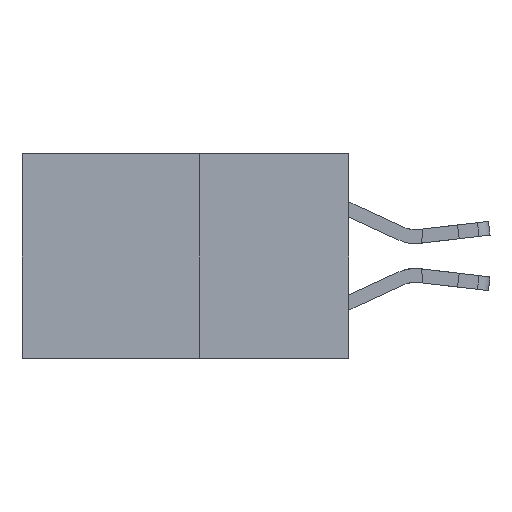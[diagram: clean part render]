
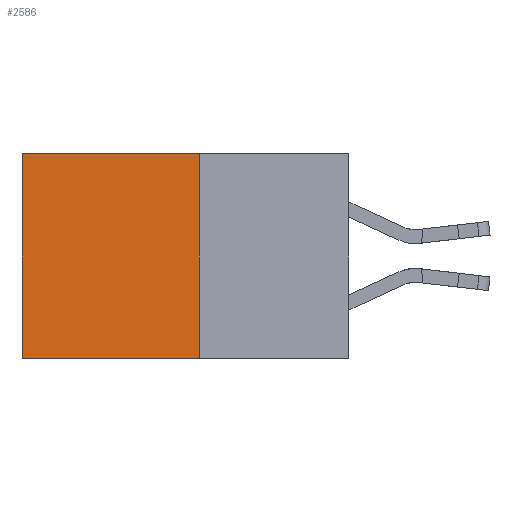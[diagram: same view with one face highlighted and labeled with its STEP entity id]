
A CAD part, left-side view. The second image highlights one B-rep face of the part: STEP entity #2586.
In plain terms, the highlighted planar face has unit normal (-1, 0, 0).
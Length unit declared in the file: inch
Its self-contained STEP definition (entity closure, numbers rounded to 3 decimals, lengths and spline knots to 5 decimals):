
#629 = VERTEX_POINT ( 'NONE', #17003 ) ;
#1297 = DIRECTION ( 'NONE',  ( 0., 1., 0. ) ) ;
#1304 = ORIENTED_EDGE ( 'NONE', *, *, #14577, .T. ) ;
#2586 = ADVANCED_FACE ( 'NONE', ( #15125 ), #15491, .F. ) ;
#3340 = DIRECTION ( 'NONE',  ( 0., 0., -1. ) ) ;
#4838 = CARTESIAN_POINT ( 'NONE',  ( 0.277, 0.27, -0.37 ) ) ;
#7273 = CARTESIAN_POINT ( 'NONE',  ( 0.277, 0.27, -0.37 ) ) ;
#7343 = CARTESIAN_POINT ( 'NONE',  ( 0.277, 0.27, -0.37 ) ) ;
#7575 = EDGE_LOOP ( 'NONE', ( #1304, #23782, #24916, #26746 ) ) ;
#7946 = CARTESIAN_POINT ( 'NONE',  ( 0.277, 0.59, -0.37 ) ) ;
#9758 = VECTOR ( 'NONE', #11988, 39.37008 ) ;
#9903 = VERTEX_POINT ( 'NONE', #7273 ) ;
#11988 = DIRECTION ( 'NONE',  ( 0., 0., -1. ) ) ;
#13415 = LINE ( 'NONE', #4838, #25134 ) ;
#13923 = LINE ( 'NONE', #26663, #19392 ) ;
#14451 = DIRECTION ( 'NONE',  ( 0., 0., -1. ) ) ;
#14547 = DIRECTION ( 'NONE',  ( 1., 0., 0. ) ) ;
#14577 = EDGE_CURVE ( 'NONE', #28130, #629, #27081, .T. ) ;
#15125 = FACE_OUTER_BOUND ( 'NONE', #7575, .T. ) ;
#15164 = CARTESIAN_POINT ( 'NONE',  ( 0.277, 0.27, -0.37 ) ) ;
#15491 = PLANE ( 'NONE',  #23619 ) ;
#16460 = EDGE_CURVE ( 'NONE', #9903, #629, #13415, .T. ) ;
#17003 = CARTESIAN_POINT ( 'NONE',  ( 0.277, 0.59, -0.37 ) ) ;
#19392 = VECTOR ( 'NONE', #22024, 39.37008 ) ;
#20809 = VECTOR ( 'NONE', #3340, 39.37008 ) ;
#22024 = DIRECTION ( 'NONE',  ( 0., 1., 0. ) ) ;
#23619 = AXIS2_PLACEMENT_3D ( 'NONE', #15164, #14547, #14451 ) ;
#23782 = ORIENTED_EDGE ( 'NONE', *, *, #16460, .F. ) ;
#24916 = ORIENTED_EDGE ( 'NONE', *, *, #30056, .F. ) ;
#25134 = VECTOR ( 'NONE', #1297, 39.37008 ) ;
#25250 = CARTESIAN_POINT ( 'NONE',  ( 0.277, 0.59, 0. ) ) ;
#26663 = CARTESIAN_POINT ( 'NONE',  ( 0.277, 0.27, 0. ) ) ;
#26746 = ORIENTED_EDGE ( 'NONE', *, *, #27191, .T. ) ;
#27081 = LINE ( 'NONE', #7946, #20809 ) ;
#27191 = EDGE_CURVE ( 'NONE', #27421, #28130, #13923, .T. ) ;
#27421 = VERTEX_POINT ( 'NONE', #27469 ) ;
#27469 = CARTESIAN_POINT ( 'NONE',  ( 0.277, 0.27, 0. ) ) ;
#28130 = VERTEX_POINT ( 'NONE', #25250 ) ;
#28455 = LINE ( 'NONE', #7343, #9758 ) ;
#30056 = EDGE_CURVE ( 'NONE', #27421, #9903, #28455, .T. ) ;
